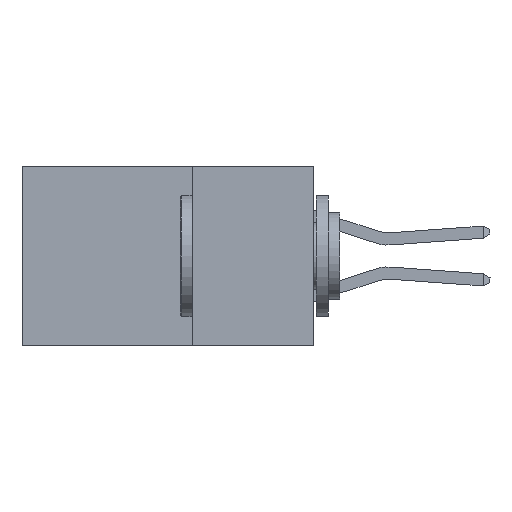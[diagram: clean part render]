
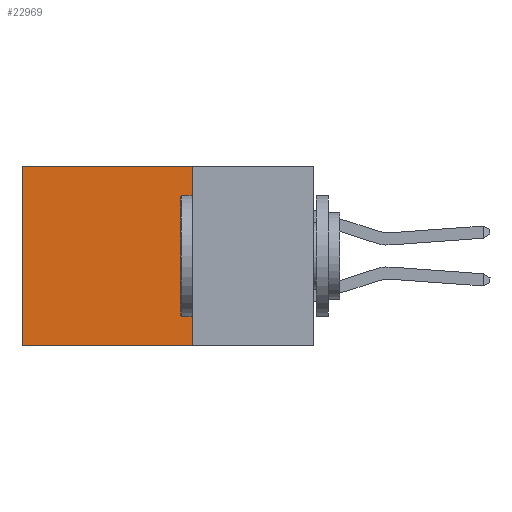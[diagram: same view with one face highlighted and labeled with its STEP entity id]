
A CAD part, left-side view. The second image highlights one B-rep face of the part: STEP entity #22969.
In plain terms, the highlighted planar face has unit normal (-1, 0, 0).
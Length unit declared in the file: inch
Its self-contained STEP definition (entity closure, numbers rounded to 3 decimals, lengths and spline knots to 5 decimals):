
#890 = AXIS2_PLACEMENT_3D ( 'NONE', #1604, #3242, #17938 ) ;
#1604 = CARTESIAN_POINT ( 'NONE',  ( 0.2875, 0.25, 0. ) ) ;
#2885 = CARTESIAN_POINT ( 'NONE',  ( 0.2875, 0.6, 0. ) ) ;
#3059 = VERTEX_POINT ( 'NONE', #24092 ) ;
#3122 = ORIENTED_EDGE ( 'NONE', *, *, #7785, .F. ) ;
#3242 = DIRECTION ( 'NONE',  ( 1., 0., 0. ) ) ;
#3328 = EDGE_CURVE ( 'NONE', #13415, #9529, #22063, .T. ) ;
#6984 = DIRECTION ( 'NONE',  ( 0., 0., -1. ) ) ;
#7139 = VERTEX_POINT ( 'NONE', #2885 ) ;
#7785 = EDGE_CURVE ( 'NONE', #9529, #3059, #23534, .T. ) ;
#8166 = EDGE_CURVE ( 'NONE', #13415, #7139, #15612, .T. ) ;
#9529 = VERTEX_POINT ( 'NONE', #14542 ) ;
#10420 = VECTOR ( 'NONE', #21800, 39.37008 ) ;
#10699 = CARTESIAN_POINT ( 'NONE',  ( 0.2875, 0.6, 0. ) ) ;
#11992 = CARTESIAN_POINT ( 'NONE',  ( 0.2875, 0.25, 0. ) ) ;
#12017 = CARTESIAN_POINT ( 'NONE',  ( 0.2875, 0.25, -0.37 ) ) ;
#13289 = PLANE ( 'NONE',  #890 ) ;
#13415 = VERTEX_POINT ( 'NONE', #15937 ) ;
#14294 = ORIENTED_EDGE ( 'NONE', *, *, #8166, .T. ) ;
#14542 = CARTESIAN_POINT ( 'NONE',  ( 0.2875, 0.25, -0.37 ) ) ;
#15021 = VECTOR ( 'NONE', #21817, 39.37008 ) ;
#15612 = LINE ( 'NONE', #11992, #10420 ) ;
#15937 = CARTESIAN_POINT ( 'NONE',  ( 0.2875, 0.25, 0. ) ) ;
#16870 = VECTOR ( 'NONE', #17253, 39.37008 ) ;
#17253 = DIRECTION ( 'NONE',  ( 0., 0., -1. ) ) ;
#17938 = DIRECTION ( 'NONE',  ( 0., 0., -1. ) ) ;
#18241 = FACE_OUTER_BOUND ( 'NONE', #18342, .T. ) ;
#18342 = EDGE_LOOP ( 'NONE', ( #24960, #3122, #19335, #14294 ) ) ;
#19335 = ORIENTED_EDGE ( 'NONE', *, *, #3328, .F. ) ;
#20747 = EDGE_CURVE ( 'NONE', #7139, #3059, #22288, .T. ) ;
#21084 = CARTESIAN_POINT ( 'NONE',  ( 0.2875, 0.25, 0. ) ) ;
#21800 = DIRECTION ( 'NONE',  ( 0., 1., 0. ) ) ;
#21817 = DIRECTION ( 'NONE',  ( 0., 1., 0. ) ) ;
#22063 = LINE ( 'NONE', #21084, #16870 ) ;
#22288 = LINE ( 'NONE', #10699, #23515 ) ;
#22969 = ADVANCED_FACE ( 'NONE', ( #18241 ), #13289, .F. ) ;
#23515 = VECTOR ( 'NONE', #6984, 39.37008 ) ;
#23534 = LINE ( 'NONE', #12017, #15021 ) ;
#24092 = CARTESIAN_POINT ( 'NONE',  ( 0.2875, 0.6, -0.37 ) ) ;
#24960 = ORIENTED_EDGE ( 'NONE', *, *, #20747, .T. ) ;
